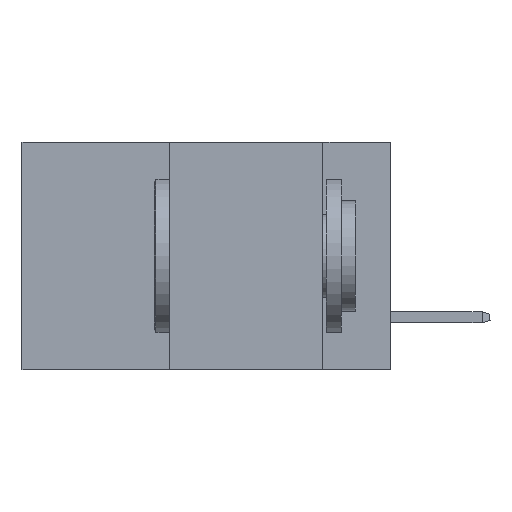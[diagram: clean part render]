
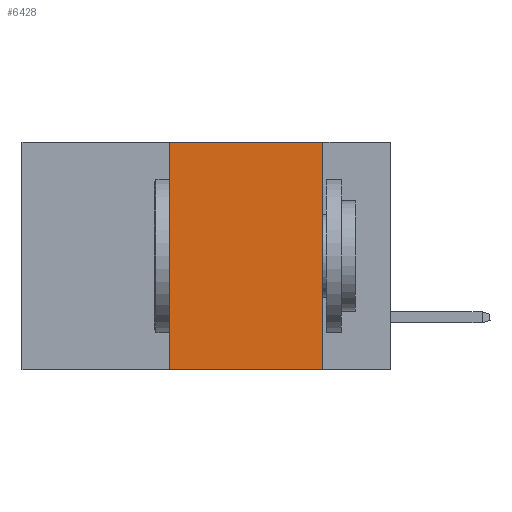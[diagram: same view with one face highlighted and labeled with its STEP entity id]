
A CAD part, left-side view. The second image highlights one B-rep face of the part: STEP entity #6428.
In plain terms, the highlighted planar face has unit normal (-1, 0, 0).
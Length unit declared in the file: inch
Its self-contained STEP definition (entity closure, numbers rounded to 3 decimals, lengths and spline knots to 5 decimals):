
#796 = VERTEX_POINT ( 'NONE', #923 ) ;
#923 = CARTESIAN_POINT ( 'NONE',  ( 0., 0.36, 0. ) ) ;
#1032 = DIRECTION ( 'NONE',  ( 0., 0., -1. ) ) ;
#1967 = DIRECTION ( 'NONE',  ( 0., 0., -1. ) ) ;
#2088 = VERTEX_POINT ( 'NONE', #3513 ) ;
#2244 = CARTESIAN_POINT ( 'NONE',  ( 0., 0.36, -0.37 ) ) ;
#2520 = VERTEX_POINT ( 'NONE', #2244 ) ;
#3199 = VERTEX_POINT ( 'NONE', #3981 ) ;
#3363 = LINE ( 'NONE', #7973, #7501 ) ;
#3490 = ORIENTED_EDGE ( 'NONE', *, *, #8064, .T. ) ;
#3513 = CARTESIAN_POINT ( 'NONE',  ( 0., 0.11, 0. ) ) ;
#3981 = CARTESIAN_POINT ( 'NONE',  ( 0., 0.11, -0.37 ) ) ;
#6428 = ADVANCED_FACE ( 'NONE', ( #12493 ), #21125, .F. ) ;
#6763 = EDGE_CURVE ( 'NONE', #2088, #3199, #14143, .T. ) ;
#7501 = VECTOR ( 'NONE', #9733, 39.37008 ) ;
#7613 = EDGE_CURVE ( 'NONE', #2520, #796, #20262, .T. ) ;
#7973 = CARTESIAN_POINT ( 'NONE',  ( 0., 0.6, 0. ) ) ;
#7981 = CARTESIAN_POINT ( 'NONE',  ( 0., 0.6, -0.37 ) ) ;
#8064 = EDGE_CURVE ( 'NONE', #2520, #3199, #20238, .T. ) ;
#8605 = CARTESIAN_POINT ( 'NONE',  ( 0., 0.36, 0. ) ) ;
#9466 = VECTOR ( 'NONE', #1032, 39.37008 ) ;
#9733 = DIRECTION ( 'NONE',  ( 0., -1., 0. ) ) ;
#9965 = VECTOR ( 'NONE', #10393, 39.37008 ) ;
#10110 = ORIENTED_EDGE ( 'NONE', *, *, #7613, .F. ) ;
#10393 = DIRECTION ( 'NONE',  ( 0., 0., 1. ) ) ;
#10819 = CARTESIAN_POINT ( 'NONE',  ( 0., 0.6, 0. ) ) ;
#11523 = DIRECTION ( 'NONE',  ( 0., -1., 0. ) ) ;
#12493 = FACE_OUTER_BOUND ( 'NONE', #13267, .T. ) ;
#12569 = DIRECTION ( 'NONE',  ( 1., 0., 0. ) ) ;
#13267 = EDGE_LOOP ( 'NONE', ( #19049, #16115, #10110, #3490 ) ) ;
#13412 = CARTESIAN_POINT ( 'NONE',  ( 0., 0.11, 0. ) ) ;
#14143 = LINE ( 'NONE', #13412, #9466 ) ;
#14618 = VECTOR ( 'NONE', #11523, 39.37008 ) ;
#15753 = EDGE_CURVE ( 'NONE', #796, #2088, #3363, .T. ) ;
#16115 = ORIENTED_EDGE ( 'NONE', *, *, #15753, .F. ) ;
#16264 = AXIS2_PLACEMENT_3D ( 'NONE', #10819, #12569, #1967 ) ;
#19049 = ORIENTED_EDGE ( 'NONE', *, *, #6763, .F. ) ;
#20238 = LINE ( 'NONE', #7981, #14618 ) ;
#20262 = LINE ( 'NONE', #8605, #9965 ) ;
#21125 = PLANE ( 'NONE',  #16264 ) ;
